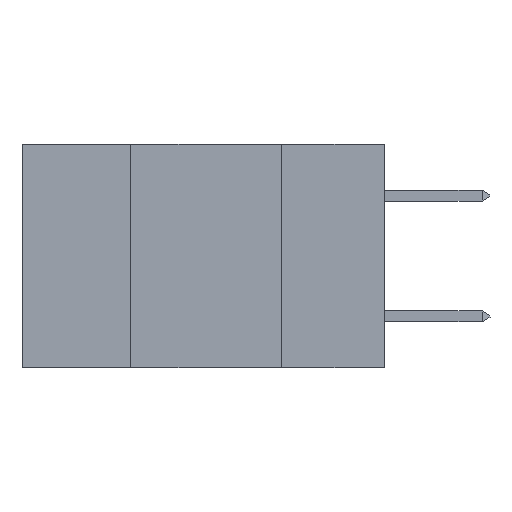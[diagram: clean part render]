
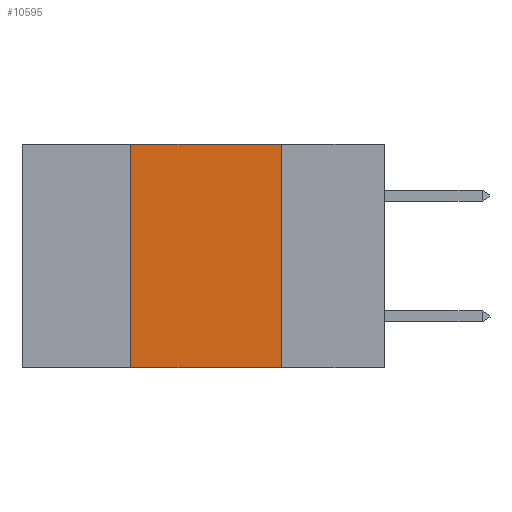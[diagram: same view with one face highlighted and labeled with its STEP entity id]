
A CAD part, left-side view. The second image highlights one B-rep face of the part: STEP entity #10595.
In plain terms, the highlighted planar face has unit normal (-1, 0, 0).
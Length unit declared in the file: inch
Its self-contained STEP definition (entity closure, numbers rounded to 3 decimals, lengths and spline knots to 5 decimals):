
#195 = CARTESIAN_POINT ( 'NONE',  ( 0., 0.42, 0. ) ) ;
#1728 = LINE ( 'NONE', #11116, #20849 ) ;
#1769 = CARTESIAN_POINT ( 'NONE',  ( 0., 0.17, 0. ) ) ;
#3033 = ORIENTED_EDGE ( 'NONE', *, *, #8622, .F. ) ;
#3304 = EDGE_CURVE ( 'NONE', #15517, #13876, #9838, .T. ) ;
#3647 = EDGE_CURVE ( 'NONE', #15517, #16819, #20670, .T. ) ;
#3944 = PLANE ( 'NONE',  #19969 ) ;
#5507 = EDGE_LOOP ( 'NONE', ( #16719, #3033, #17870, #23188 ) ) ;
#5853 = EDGE_CURVE ( 'NONE', #18297, #16819, #22636, .T. ) ;
#6585 = VECTOR ( 'NONE', #18359, 39.37008 ) ;
#7425 = DIRECTION ( 'NONE',  ( 0., 0., -1. ) ) ;
#8242 = CARTESIAN_POINT ( 'NONE',  ( 0., 0.42, 0. ) ) ;
#8622 = EDGE_CURVE ( 'NONE', #13876, #18297, #1728, .T. ) ;
#9610 = CARTESIAN_POINT ( 'NONE',  ( 0., 0.6, 0. ) ) ;
#9838 = LINE ( 'NONE', #8242, #18991 ) ;
#10595 = ADVANCED_FACE ( 'NONE', ( #12040 ), #3944, .F. ) ;
#11116 = CARTESIAN_POINT ( 'NONE',  ( 0., 0.6, 0. ) ) ;
#11430 = DIRECTION ( 'NONE',  ( 0., 0., -1. ) ) ;
#12040 = FACE_OUTER_BOUND ( 'NONE', #5507, .T. ) ;
#12973 = VECTOR ( 'NONE', #7425, 39.37008 ) ;
#13876 = VERTEX_POINT ( 'NONE', #195 ) ;
#15142 = CARTESIAN_POINT ( 'NONE',  ( 0., 0.17, -0.37 ) ) ;
#15517 = VERTEX_POINT ( 'NONE', #23265 ) ;
#15645 = DIRECTION ( 'NONE',  ( 0., 0., 1. ) ) ;
#16526 = CARTESIAN_POINT ( 'NONE',  ( 0., 0.6, -0.37 ) ) ;
#16719 = ORIENTED_EDGE ( 'NONE', *, *, #5853, .F. ) ;
#16819 = VERTEX_POINT ( 'NONE', #15142 ) ;
#17870 = ORIENTED_EDGE ( 'NONE', *, *, #3304, .F. ) ;
#18297 = VERTEX_POINT ( 'NONE', #23069 ) ;
#18359 = DIRECTION ( 'NONE',  ( 0., -1., 0. ) ) ;
#18991 = VECTOR ( 'NONE', #15645, 39.37008 ) ;
#19969 = AXIS2_PLACEMENT_3D ( 'NONE', #9610, #22326, #11430 ) ;
#20670 = LINE ( 'NONE', #16526, #6585 ) ;
#20849 = VECTOR ( 'NONE', #22091, 39.37008 ) ;
#22091 = DIRECTION ( 'NONE',  ( 0., -1., 0. ) ) ;
#22326 = DIRECTION ( 'NONE',  ( 1., 0., 0. ) ) ;
#22636 = LINE ( 'NONE', #1769, #12973 ) ;
#23069 = CARTESIAN_POINT ( 'NONE',  ( 0., 0.17, 0. ) ) ;
#23188 = ORIENTED_EDGE ( 'NONE', *, *, #3647, .T. ) ;
#23265 = CARTESIAN_POINT ( 'NONE',  ( 0., 0.42, -0.37 ) ) ;
